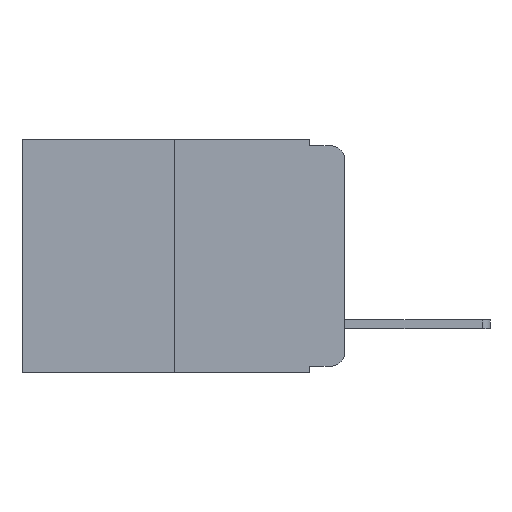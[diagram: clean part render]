
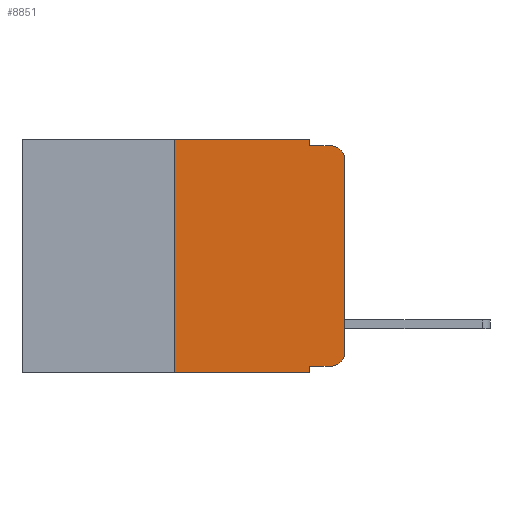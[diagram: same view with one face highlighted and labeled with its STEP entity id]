
A CAD part, left-side view. The second image highlights one B-rep face of the part: STEP entity #8851.
In plain terms, the highlighted planar face has unit normal (-1, 0, 0).
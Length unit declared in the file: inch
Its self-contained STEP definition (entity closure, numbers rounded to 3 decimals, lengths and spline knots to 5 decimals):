
#103 = LINE ( 'NONE', #5120, #2894 ) ;
#581 = EDGE_CURVE ( 'NONE', #4864, #8464, #15628, .T. ) ;
#1165 = ORIENTED_EDGE ( 'NONE', *, *, #8160, .F. ) ;
#1439 = LINE ( 'NONE', #4768, #14117 ) ;
#1615 = CARTESIAN_POINT ( 'NONE',  ( 0., 0.02, -0.313 ) ) ;
#1684 = CARTESIAN_POINT ( 'NONE',  ( 0., 0.051, 0. ) ) ;
#1779 = ORIENTED_EDGE ( 'NONE', *, *, #6135, .T. ) ;
#1953 = VERTEX_POINT ( 'NONE', #1684 ) ;
#2268 = VECTOR ( 'NONE', #17290, 39.37008 ) ;
#2289 = DIRECTION ( 'NONE',  ( 0., 0., -1. ) ) ;
#2357 = CARTESIAN_POINT ( 'NONE',  ( 0., 0.02, -0.01 ) ) ;
#2876 = ORIENTED_EDGE ( 'NONE', *, *, #581, .F. ) ;
#2877 = EDGE_LOOP ( 'NONE', ( #1779, #13433, #16898, #13857, #15072, #1165, #15480, #2876, #6474, #3294 ) ) ;
#2894 = VECTOR ( 'NONE', #6964, 39.37008 ) ;
#3002 = DIRECTION ( 'NONE',  ( 0., 0., -1. ) ) ;
#3058 = AXIS2_PLACEMENT_3D ( 'NONE', #10380, #10486, #8903 ) ;
#3294 = ORIENTED_EDGE ( 'NONE', *, *, #11045, .T. ) ;
#3348 = EDGE_CURVE ( 'NONE', #8186, #8464, #4261, .T. ) ;
#4261 = LINE ( 'NONE', #4515, #11891 ) ;
#4284 = DIRECTION ( 'NONE',  ( -1., 0., 0. ) ) ;
#4298 = CARTESIAN_POINT ( 'NONE',  ( 0., 0.02, -0.03 ) ) ;
#4363 = VERTEX_POINT ( 'NONE', #2357 ) ;
#4375 = LINE ( 'NONE', #13247, #14711 ) ;
#4475 = DIRECTION ( 'NONE',  ( 0., -1., 0. ) ) ;
#4515 = CARTESIAN_POINT ( 'NONE',  ( 0., 0.473, -0.343 ) ) ;
#4595 = CIRCLE ( 'NONE', #12183, 0.02 ) ;
#4768 = CARTESIAN_POINT ( 'NONE',  ( 0., 0.25, 0. ) ) ;
#4787 = CARTESIAN_POINT ( 'NONE',  ( 0., 0.02, -0.333 ) ) ;
#4864 = VERTEX_POINT ( 'NONE', #10685 ) ;
#5120 = CARTESIAN_POINT ( 'NONE',  ( 0., 0.051, -0.333 ) ) ;
#5517 = EDGE_CURVE ( 'NONE', #14293, #4363, #4595, .T. ) ;
#5536 = LINE ( 'NONE', #8953, #8722 ) ;
#5853 = DIRECTION ( 'NONE',  ( 0., 0., -1. ) ) ;
#6051 = CARTESIAN_POINT ( 'NONE',  ( 0., 0.051, 0. ) ) ;
#6135 = EDGE_CURVE ( 'NONE', #15281, #14293, #9864, .T. ) ;
#6473 = EDGE_CURVE ( 'NONE', #8590, #1953, #4375, .T. ) ;
#6474 = ORIENTED_EDGE ( 'NONE', *, *, #9077, .T. ) ;
#6720 = FACE_OUTER_BOUND ( 'NONE', #2877, .T. ) ;
#6927 = VERTEX_POINT ( 'NONE', #4787 ) ;
#6964 = DIRECTION ( 'NONE',  ( 0., -1., 0. ) ) ;
#7985 = CARTESIAN_POINT ( 'NONE',  ( 0., 0.051, -0.01 ) ) ;
#8009 = DIRECTION ( 'NONE',  ( 0., -1., 0. ) ) ;
#8160 = EDGE_CURVE ( 'NONE', #8186, #8590, #1439, .T. ) ;
#8186 = VERTEX_POINT ( 'NONE', #11984 ) ;
#8464 = VERTEX_POINT ( 'NONE', #11296 ) ;
#8590 = VERTEX_POINT ( 'NONE', #15924 ) ;
#8722 = VECTOR ( 'NONE', #13035, 39.37008 ) ;
#8851 = ADVANCED_FACE ( 'NONE', ( #6720 ), #11749, .F. ) ;
#8869 = AXIS2_PLACEMENT_3D ( 'NONE', #1615, #11092, #3002 ) ;
#8879 = EDGE_CURVE ( 'NONE', #9879, #4363, #13062, .T. ) ;
#8903 = DIRECTION ( 'NONE',  ( 0., 0., -1. ) ) ;
#8953 = CARTESIAN_POINT ( 'NONE',  ( 0., 0.051, 0. ) ) ;
#9077 = EDGE_CURVE ( 'NONE', #4864, #6927, #103, .T. ) ;
#9864 = LINE ( 'NONE', #17306, #2268 ) ;
#9879 = VERTEX_POINT ( 'NONE', #11202 ) ;
#10380 = CARTESIAN_POINT ( 'NONE',  ( 0., 0.473, 0. ) ) ;
#10486 = DIRECTION ( 'NONE',  ( 1., 0., 0. ) ) ;
#10685 = CARTESIAN_POINT ( 'NONE',  ( 0., 0.051, -0.333 ) ) ;
#11045 = EDGE_CURVE ( 'NONE', #6927, #15281, #12982, .T. ) ;
#11092 = DIRECTION ( 'NONE',  ( -1., 0., 0. ) ) ;
#11202 = CARTESIAN_POINT ( 'NONE',  ( 0., 0.051, -0.01 ) ) ;
#11296 = CARTESIAN_POINT ( 'NONE',  ( 0., 0.051, -0.343 ) ) ;
#11749 = PLANE ( 'NONE',  #3058 ) ;
#11891 = VECTOR ( 'NONE', #4475, 39.37008 ) ;
#11984 = CARTESIAN_POINT ( 'NONE',  ( 0., 0.25, -0.343 ) ) ;
#12138 = VECTOR ( 'NONE', #5853, 39.37008 ) ;
#12183 = AXIS2_PLACEMENT_3D ( 'NONE', #4298, #4284, #2289 ) ;
#12982 = CIRCLE ( 'NONE', #8869, 0.02 ) ;
#13035 = DIRECTION ( 'NONE',  ( 0., 0., -1. ) ) ;
#13062 = LINE ( 'NONE', #7985, #16118 ) ;
#13212 = DIRECTION ( 'NONE',  ( 0., -1., 0. ) ) ;
#13247 = CARTESIAN_POINT ( 'NONE',  ( 0., 0.473, 0. ) ) ;
#13433 = ORIENTED_EDGE ( 'NONE', *, *, #5517, .T. ) ;
#13857 = ORIENTED_EDGE ( 'NONE', *, *, #16212, .F. ) ;
#14117 = VECTOR ( 'NONE', #16110, 39.37008 ) ;
#14128 = CARTESIAN_POINT ( 'NONE',  ( 0., 0., -0.03 ) ) ;
#14293 = VERTEX_POINT ( 'NONE', #14128 ) ;
#14711 = VECTOR ( 'NONE', #13212, 39.37008 ) ;
#14896 = CARTESIAN_POINT ( 'NONE',  ( 0., 0., -0.313 ) ) ;
#15072 = ORIENTED_EDGE ( 'NONE', *, *, #6473, .F. ) ;
#15281 = VERTEX_POINT ( 'NONE', #14896 ) ;
#15480 = ORIENTED_EDGE ( 'NONE', *, *, #3348, .T. ) ;
#15628 = LINE ( 'NONE', #6051, #12138 ) ;
#15924 = CARTESIAN_POINT ( 'NONE',  ( 0., 0.25, 0. ) ) ;
#16110 = DIRECTION ( 'NONE',  ( 0., 0., 1. ) ) ;
#16118 = VECTOR ( 'NONE', #8009, 39.37008 ) ;
#16212 = EDGE_CURVE ( 'NONE', #1953, #9879, #5536, .T. ) ;
#16898 = ORIENTED_EDGE ( 'NONE', *, *, #8879, .F. ) ;
#17290 = DIRECTION ( 'NONE',  ( 0., 0., 1. ) ) ;
#17306 = CARTESIAN_POINT ( 'NONE',  ( 0., 0., 0. ) ) ;
